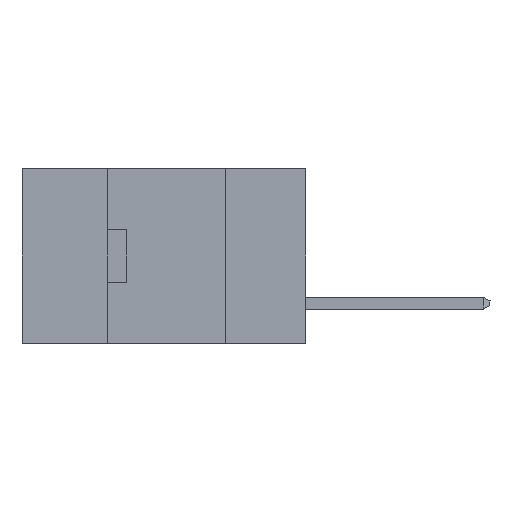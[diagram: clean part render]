
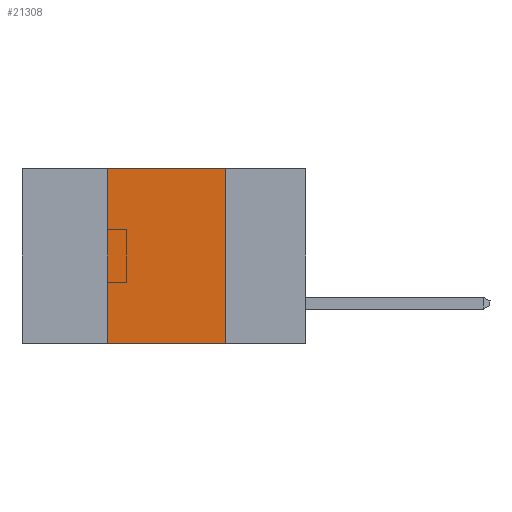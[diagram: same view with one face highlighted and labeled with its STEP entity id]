
A CAD part, left-side view. The second image highlights one B-rep face of the part: STEP entity #21308.
In plain terms, the highlighted planar face has unit normal (-1, 0, 0).
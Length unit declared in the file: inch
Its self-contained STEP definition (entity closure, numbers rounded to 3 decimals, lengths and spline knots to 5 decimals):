
#343 = CARTESIAN_POINT ( 'NONE',  ( 0., 0.6, 0. ) ) ;
#892 = DIRECTION ( 'NONE',  ( 0., 0., 1. ) ) ;
#1195 = VECTOR ( 'NONE', #20567, 39.37008 ) ;
#3204 = VERTEX_POINT ( 'NONE', #6946 ) ;
#4137 = LINE ( 'NONE', #12484, #13548 ) ;
#6492 = DIRECTION ( 'NONE',  ( 0., 0., -1. ) ) ;
#6723 = CARTESIAN_POINT ( 'NONE',  ( 0., 0.17, -0.37 ) ) ;
#6946 = CARTESIAN_POINT ( 'NONE',  ( 0., 0.42, 0. ) ) ;
#7277 = CARTESIAN_POINT ( 'NONE',  ( 0., 0.6, 0. ) ) ;
#7332 = LINE ( 'NONE', #13073, #21617 ) ;
#8255 = EDGE_CURVE ( 'NONE', #10924, #15542, #4137, .T. ) ;
#9691 = ORIENTED_EDGE ( 'NONE', *, *, #20344, .F. ) ;
#10477 = DIRECTION ( 'NONE',  ( 1., 0., 0. ) ) ;
#10924 = VERTEX_POINT ( 'NONE', #18837 ) ;
#11014 = PLANE ( 'NONE',  #17042 ) ;
#12484 = CARTESIAN_POINT ( 'NONE',  ( 0., 0.6, -0.37 ) ) ;
#13008 = ORIENTED_EDGE ( 'NONE', *, *, #8255, .T. ) ;
#13073 = CARTESIAN_POINT ( 'NONE',  ( 0., 0.42, -0.37 ) ) ;
#13548 = VECTOR ( 'NONE', #19336, 39.37008 ) ;
#14910 = VERTEX_POINT ( 'NONE', #15993 ) ;
#15253 = EDGE_CURVE ( 'NONE', #10924, #3204, #7332, .T. ) ;
#15542 = VERTEX_POINT ( 'NONE', #6723 ) ;
#15993 = CARTESIAN_POINT ( 'NONE',  ( 0., 0.17, 0. ) ) ;
#17042 = AXIS2_PLACEMENT_3D ( 'NONE', #343, #10477, #6492 ) ;
#18476 = VECTOR ( 'NONE', #19204, 39.37008 ) ;
#18824 = FACE_OUTER_BOUND ( 'NONE', #24447, .T. ) ;
#18837 = CARTESIAN_POINT ( 'NONE',  ( 0., 0.42, -0.37 ) ) ;
#19204 = DIRECTION ( 'NONE',  ( 0., -1., 0. ) ) ;
#19336 = DIRECTION ( 'NONE',  ( 0., -1., 0. ) ) ;
#20162 = LINE ( 'NONE', #24659, #1195 ) ;
#20164 = ORIENTED_EDGE ( 'NONE', *, *, #26787, .F. ) ;
#20344 = EDGE_CURVE ( 'NONE', #14910, #15542, #20162, .T. ) ;
#20567 = DIRECTION ( 'NONE',  ( 0., 0., -1. ) ) ;
#21308 = ADVANCED_FACE ( 'NONE', ( #18824 ), #11014, .F. ) ;
#21617 = VECTOR ( 'NONE', #892, 39.37008 ) ;
#21660 = LINE ( 'NONE', #7277, #18476 ) ;
#24447 = EDGE_LOOP ( 'NONE', ( #9691, #20164, #26014, #13008 ) ) ;
#24659 = CARTESIAN_POINT ( 'NONE',  ( 0., 0.17, -0.37 ) ) ;
#26014 = ORIENTED_EDGE ( 'NONE', *, *, #15253, .F. ) ;
#26787 = EDGE_CURVE ( 'NONE', #3204, #14910, #21660, .T. ) ;
